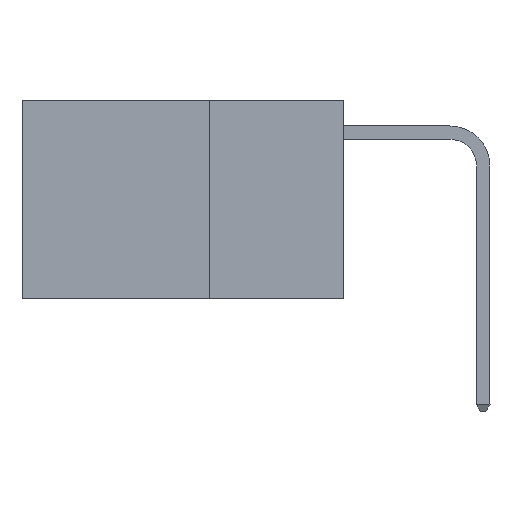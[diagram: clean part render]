
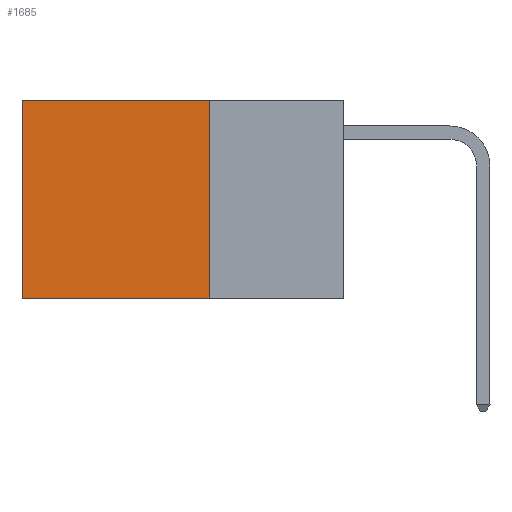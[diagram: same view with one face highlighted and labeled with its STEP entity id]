
A CAD part, left-side view. The second image highlights one B-rep face of the part: STEP entity #1685.
In plain terms, the highlighted planar face has unit normal (-1, 0, 0).
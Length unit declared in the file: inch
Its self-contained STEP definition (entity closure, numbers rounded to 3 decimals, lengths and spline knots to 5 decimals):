
#369 = EDGE_LOOP ( 'NONE', ( #11919, #13483, #17065, #4945 ) ) ;
#442 = CARTESIAN_POINT ( 'NONE',  ( 0.2625, 0.6, 0. ) ) ;
#1685 = ADVANCED_FACE ( 'NONE', ( #9364 ), #8035, .F. ) ;
#1783 = VECTOR ( 'NONE', #15626, 39.37008 ) ;
#1908 = EDGE_CURVE ( 'NONE', #15968, #15290, #11698, .T. ) ;
#2366 = LINE ( 'NONE', #3700, #15983 ) ;
#2423 = EDGE_CURVE ( 'NONE', #15290, #2469, #2366, .T. ) ;
#2469 = VERTEX_POINT ( 'NONE', #7818 ) ;
#3700 = CARTESIAN_POINT ( 'NONE',  ( 0.2625, 0.6, 0. ) ) ;
#3756 = EDGE_CURVE ( 'NONE', #15968, #14951, #4925, .T. ) ;
#3790 = DIRECTION ( 'NONE',  ( 0., 0., -1. ) ) ;
#3809 = DIRECTION ( 'NONE',  ( 0., 1., 0. ) ) ;
#4255 = DIRECTION ( 'NONE',  ( 0., 0., -1. ) ) ;
#4925 = LINE ( 'NONE', #10287, #1783 ) ;
#4945 = ORIENTED_EDGE ( 'NONE', *, *, #1908, .T. ) ;
#7385 = VECTOR ( 'NONE', #14442, 39.37008 ) ;
#7818 = CARTESIAN_POINT ( 'NONE',  ( 0.2625, 0.6, -0.37 ) ) ;
#8035 = PLANE ( 'NONE',  #13040 ) ;
#8613 = VECTOR ( 'NONE', #3809, 39.37008 ) ;
#9364 = FACE_OUTER_BOUND ( 'NONE', #369, .T. ) ;
#10287 = CARTESIAN_POINT ( 'NONE',  ( 0.2625, 0.25, 0. ) ) ;
#11698 = LINE ( 'NONE', #15819, #8613 ) ;
#11736 = CARTESIAN_POINT ( 'NONE',  ( 0.2625, 0.25, -0.37 ) ) ;
#11919 = ORIENTED_EDGE ( 'NONE', *, *, #2423, .T. ) ;
#13040 = AXIS2_PLACEMENT_3D ( 'NONE', #16276, #14687, #4255 ) ;
#13047 = LINE ( 'NONE', #11736, #7385 ) ;
#13483 = ORIENTED_EDGE ( 'NONE', *, *, #16048, .F. ) ;
#14442 = DIRECTION ( 'NONE',  ( 0., 1., 0. ) ) ;
#14687 = DIRECTION ( 'NONE',  ( 1., 0., 0. ) ) ;
#14951 = VERTEX_POINT ( 'NONE', #16696 ) ;
#15290 = VERTEX_POINT ( 'NONE', #442 ) ;
#15626 = DIRECTION ( 'NONE',  ( 0., 0., -1. ) ) ;
#15819 = CARTESIAN_POINT ( 'NONE',  ( 0.2625, 0.25, 0. ) ) ;
#15968 = VERTEX_POINT ( 'NONE', #16910 ) ;
#15983 = VECTOR ( 'NONE', #3790, 39.37008 ) ;
#16048 = EDGE_CURVE ( 'NONE', #14951, #2469, #13047, .T. ) ;
#16276 = CARTESIAN_POINT ( 'NONE',  ( 0.2625, 0.25, 0. ) ) ;
#16696 = CARTESIAN_POINT ( 'NONE',  ( 0.2625, 0.25, -0.37 ) ) ;
#16910 = CARTESIAN_POINT ( 'NONE',  ( 0.2625, 0.25, 0. ) ) ;
#17065 = ORIENTED_EDGE ( 'NONE', *, *, #3756, .F. ) ;
